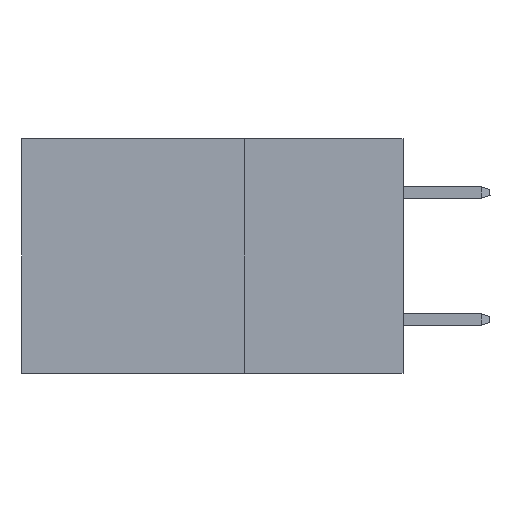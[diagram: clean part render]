
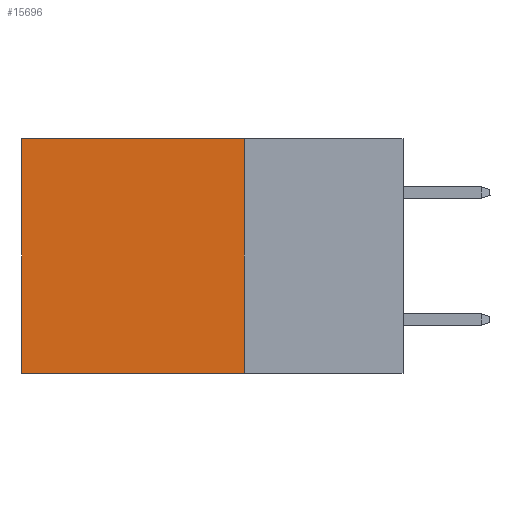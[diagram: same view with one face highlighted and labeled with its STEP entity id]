
A CAD part, left-side view. The second image highlights one B-rep face of the part: STEP entity #15696.
In plain terms, the highlighted planar face has unit normal (-1, 0, 0).
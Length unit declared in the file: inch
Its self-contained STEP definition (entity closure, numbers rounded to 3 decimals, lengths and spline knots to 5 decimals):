
#2106 = ORIENTED_EDGE ( 'NONE', *, *, #18340, .F. ) ;
#2798 = VECTOR ( 'NONE', #22946, 39.37008 ) ;
#3506 = CARTESIAN_POINT ( 'NONE',  ( 0.2875, 0.6, 0. ) ) ;
#4257 = LINE ( 'NONE', #14449, #32816 ) ;
#10814 = CARTESIAN_POINT ( 'NONE',  ( 0.2875, 0.25, 0. ) ) ;
#11414 = EDGE_CURVE ( 'NONE', #42270, #37179, #4257, .T. ) ;
#12228 = EDGE_CURVE ( 'NONE', #37179, #26021, #40131, .T. ) ;
#13728 = LINE ( 'NONE', #30245, #36459 ) ;
#14161 = ORIENTED_EDGE ( 'NONE', *, *, #12228, .T. ) ;
#14449 = CARTESIAN_POINT ( 'NONE',  ( 0.2875, 0.25, 0. ) ) ;
#15696 = ADVANCED_FACE ( 'NONE', ( #33630 ), #30180, .F. ) ;
#15848 = CARTESIAN_POINT ( 'NONE',  ( 0.2875, 0.6, 0. ) ) ;
#16009 = LINE ( 'NONE', #29266, #2798 ) ;
#17346 = CARTESIAN_POINT ( 'NONE',  ( 0.2875, 0.25, 0. ) ) ;
#18340 = EDGE_CURVE ( 'NONE', #30026, #26021, #13728, .T. ) ;
#19580 = VECTOR ( 'NONE', #27741, 39.37008 ) ;
#22174 = CARTESIAN_POINT ( 'NONE',  ( 0.2875, 0.6, -0.37 ) ) ;
#22946 = DIRECTION ( 'NONE',  ( 0., 0., -1. ) ) ;
#26021 = VERTEX_POINT ( 'NONE', #22174 ) ;
#27741 = DIRECTION ( 'NONE',  ( 0., 0., -1. ) ) ;
#29194 = EDGE_CURVE ( 'NONE', #42270, #30026, #16009, .T. ) ;
#29266 = CARTESIAN_POINT ( 'NONE',  ( 0.2875, 0.25, 0. ) ) ;
#29510 = AXIS2_PLACEMENT_3D ( 'NONE', #17346, #30610, #40753 ) ;
#30026 = VERTEX_POINT ( 'NONE', #36850 ) ;
#30180 = PLANE ( 'NONE',  #29510 ) ;
#30245 = CARTESIAN_POINT ( 'NONE',  ( 0.2875, 0.25, -0.37 ) ) ;
#30610 = DIRECTION ( 'NONE',  ( 1., 0., 0. ) ) ;
#31305 = EDGE_LOOP ( 'NONE', ( #14161, #2106, #32511, #31498 ) ) ;
#31498 = ORIENTED_EDGE ( 'NONE', *, *, #11414, .T. ) ;
#32511 = ORIENTED_EDGE ( 'NONE', *, *, #29194, .F. ) ;
#32816 = VECTOR ( 'NONE', #34410, 39.37008 ) ;
#33630 = FACE_OUTER_BOUND ( 'NONE', #31305, .T. ) ;
#34410 = DIRECTION ( 'NONE',  ( 0., 1., 0. ) ) ;
#36459 = VECTOR ( 'NONE', #36926, 39.37008 ) ;
#36850 = CARTESIAN_POINT ( 'NONE',  ( 0.2875, 0.25, -0.37 ) ) ;
#36926 = DIRECTION ( 'NONE',  ( 0., 1., 0. ) ) ;
#37179 = VERTEX_POINT ( 'NONE', #15848 ) ;
#40131 = LINE ( 'NONE', #3506, #19580 ) ;
#40753 = DIRECTION ( 'NONE',  ( 0., 0., -1. ) ) ;
#42270 = VERTEX_POINT ( 'NONE', #10814 ) ;
